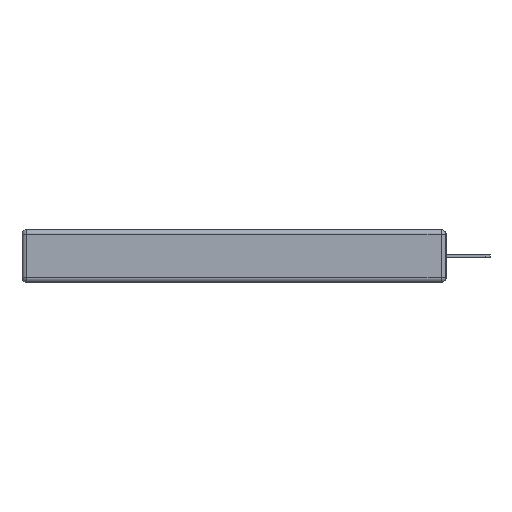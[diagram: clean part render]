
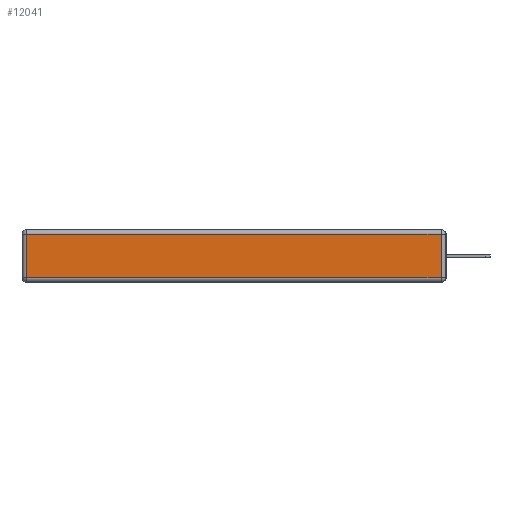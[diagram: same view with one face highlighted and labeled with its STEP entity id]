
A CAD part, left-side view. The second image highlights one B-rep face of the part: STEP entity #12041.
In plain terms, the highlighted planar face has unit normal (-1, 0, 0).
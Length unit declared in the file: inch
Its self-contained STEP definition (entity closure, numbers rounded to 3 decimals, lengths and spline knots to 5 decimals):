
#445 = DIRECTION ( 'NONE',  ( 0., 1., 0. ) ) ;
#1381 = CARTESIAN_POINT ( 'NONE',  ( 0., 2.72, -0.03 ) ) ;
#1503 = ORIENTED_EDGE ( 'NONE', *, *, #11016, .T. ) ;
#1619 = ORIENTED_EDGE ( 'NONE', *, *, #4497, .T. ) ;
#1660 = VECTOR ( 'NONE', #12853, 39.37008 ) ;
#2488 = CARTESIAN_POINT ( 'NONE',  ( 0., 0., -0.343 ) ) ;
#2928 = DIRECTION ( 'NONE',  ( 0., 0., 1. ) ) ;
#3865 = DIRECTION ( 'NONE',  ( 0., -1., 0. ) ) ;
#4497 = EDGE_CURVE ( 'NONE', #10210, #6046, #11171, .T. ) ;
#4727 = VERTEX_POINT ( 'NONE', #6177 ) ;
#4840 = FACE_OUTER_BOUND ( 'NONE', #14931, .T. ) ;
#5813 = ORIENTED_EDGE ( 'NONE', *, *, #13392, .T. ) ;
#6046 = VERTEX_POINT ( 'NONE', #1381 ) ;
#6177 = CARTESIAN_POINT ( 'NONE',  ( 0., 2.72, -0.313 ) ) ;
#6974 = EDGE_CURVE ( 'NONE', #6046, #4727, #11588, .T. ) ;
#7063 = PLANE ( 'NONE',  #14673 ) ;
#7978 = ORIENTED_EDGE ( 'NONE', *, *, #6974, .T. ) ;
#8945 = VECTOR ( 'NONE', #445, 39.37008 ) ;
#10210 = VERTEX_POINT ( 'NONE', #10424 ) ;
#10424 = CARTESIAN_POINT ( 'NONE',  ( 0., 0.03, -0.03 ) ) ;
#11016 = EDGE_CURVE ( 'NONE', #14166, #10210, #12498, .T. ) ;
#11092 = VECTOR ( 'NONE', #2928, 39.37008 ) ;
#11100 = CARTESIAN_POINT ( 'NONE',  ( 0., 0., -0.313 ) ) ;
#11171 = LINE ( 'NONE', #13723, #8945 ) ;
#11588 = LINE ( 'NONE', #12693, #1660 ) ;
#12041 = ADVANCED_FACE ( 'NONE', ( #4840 ), #7063, .T. ) ;
#12059 = DIRECTION ( 'NONE',  ( -1., 0., 0. ) ) ;
#12366 = LINE ( 'NONE', #11100, #13711 ) ;
#12498 = LINE ( 'NONE', #14880, #11092 ) ;
#12693 = CARTESIAN_POINT ( 'NONE',  ( 0., 2.72, -0.343 ) ) ;
#12853 = DIRECTION ( 'NONE',  ( 0., 0., -1. ) ) ;
#13175 = DIRECTION ( 'NONE',  ( 0., 0., 1. ) ) ;
#13392 = EDGE_CURVE ( 'NONE', #4727, #14166, #12366, .T. ) ;
#13711 = VECTOR ( 'NONE', #3865, 39.37008 ) ;
#13723 = CARTESIAN_POINT ( 'NONE',  ( 0., 2.75, -0.03 ) ) ;
#14166 = VERTEX_POINT ( 'NONE', #15589 ) ;
#14673 = AXIS2_PLACEMENT_3D ( 'NONE', #2488, #12059, #13175 ) ;
#14880 = CARTESIAN_POINT ( 'NONE',  ( 0., 0.03, -0.343 ) ) ;
#14931 = EDGE_LOOP ( 'NONE', ( #5813, #1503, #1619, #7978 ) ) ;
#15589 = CARTESIAN_POINT ( 'NONE',  ( 0., 0.03, -0.313 ) ) ;
